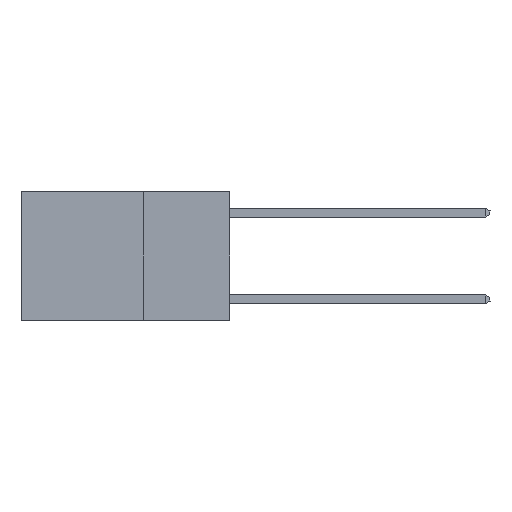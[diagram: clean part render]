
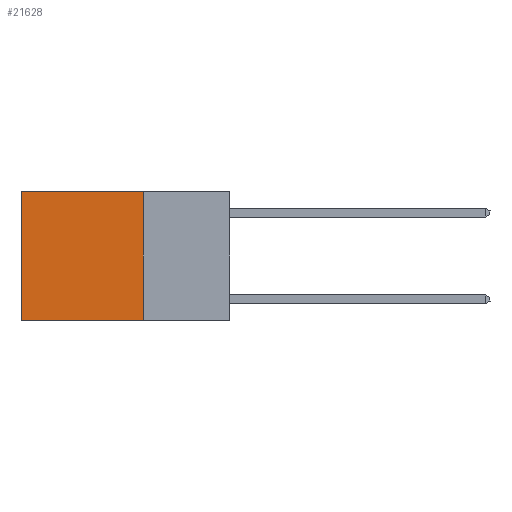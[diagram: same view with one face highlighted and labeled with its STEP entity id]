
A CAD part, left-side view. The second image highlights one B-rep face of the part: STEP entity #21628.
In plain terms, the highlighted planar face has unit normal (-1, 0, 0).
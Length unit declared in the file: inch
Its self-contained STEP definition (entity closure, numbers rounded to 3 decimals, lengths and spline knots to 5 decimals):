
#1017 = CARTESIAN_POINT ( 'NONE',  ( 0.2625, 0.25, 0. ) ) ;
#1842 = CARTESIAN_POINT ( 'NONE',  ( 0.2625, 0.6, 0. ) ) ;
#2047 = VERTEX_POINT ( 'NONE', #1017 ) ;
#2718 = VERTEX_POINT ( 'NONE', #6533 ) ;
#3231 = VERTEX_POINT ( 'NONE', #1842 ) ;
#3977 = CARTESIAN_POINT ( 'NONE',  ( 0.2625, 0.25, -0.37 ) ) ;
#4500 = EDGE_CURVE ( 'NONE', #2718, #26613, #28394, .T. ) ;
#5030 = CARTESIAN_POINT ( 'NONE',  ( 0.2625, 0.25, 0. ) ) ;
#6533 = CARTESIAN_POINT ( 'NONE',  ( 0.2625, 0.25, -0.37 ) ) ;
#7472 = EDGE_LOOP ( 'NONE', ( #25887, #17230, #28754, #27053 ) ) ;
#8342 = CARTESIAN_POINT ( 'NONE',  ( 0.2625, 0.25, 0. ) ) ;
#8467 = CARTESIAN_POINT ( 'NONE',  ( 0.2625, 0.6, 0. ) ) ;
#10338 = LINE ( 'NONE', #29786, #12474 ) ;
#12474 = VECTOR ( 'NONE', #18639, 39.37008 ) ;
#12975 = LINE ( 'NONE', #8342, #31387 ) ;
#13887 = DIRECTION ( 'NONE',  ( 0., 1., 0. ) ) ;
#17230 = ORIENTED_EDGE ( 'NONE', *, *, #4500, .F. ) ;
#17376 = EDGE_CURVE ( 'NONE', #3231, #26613, #21235, .T. ) ;
#18196 = AXIS2_PLACEMENT_3D ( 'NONE', #5030, #28668, #24051 ) ;
#18209 = DIRECTION ( 'NONE',  ( 0., 0., -1. ) ) ;
#18639 = DIRECTION ( 'NONE',  ( 0., 0., -1. ) ) ;
#20862 = VECTOR ( 'NONE', #13887, 39.37008 ) ;
#21006 = EDGE_CURVE ( 'NONE', #2047, #3231, #12975, .T. ) ;
#21235 = LINE ( 'NONE', #8467, #28667 ) ;
#21628 = ADVANCED_FACE ( 'NONE', ( #26306 ), #26759, .F. ) ;
#22698 = DIRECTION ( 'NONE',  ( 0., 1., 0. ) ) ;
#24051 = DIRECTION ( 'NONE',  ( 0., 0., -1. ) ) ;
#25352 = CARTESIAN_POINT ( 'NONE',  ( 0.2625, 0.6, -0.37 ) ) ;
#25887 = ORIENTED_EDGE ( 'NONE', *, *, #17376, .T. ) ;
#26306 = FACE_OUTER_BOUND ( 'NONE', #7472, .T. ) ;
#26600 = EDGE_CURVE ( 'NONE', #2047, #2718, #10338, .T. ) ;
#26613 = VERTEX_POINT ( 'NONE', #25352 ) ;
#26759 = PLANE ( 'NONE',  #18196 ) ;
#27053 = ORIENTED_EDGE ( 'NONE', *, *, #21006, .T. ) ;
#28394 = LINE ( 'NONE', #3977, #20862 ) ;
#28667 = VECTOR ( 'NONE', #18209, 39.37008 ) ;
#28668 = DIRECTION ( 'NONE',  ( 1., 0., 0. ) ) ;
#28754 = ORIENTED_EDGE ( 'NONE', *, *, #26600, .F. ) ;
#29786 = CARTESIAN_POINT ( 'NONE',  ( 0.2625, 0.25, 0. ) ) ;
#31387 = VECTOR ( 'NONE', #22698, 39.37008 ) ;
